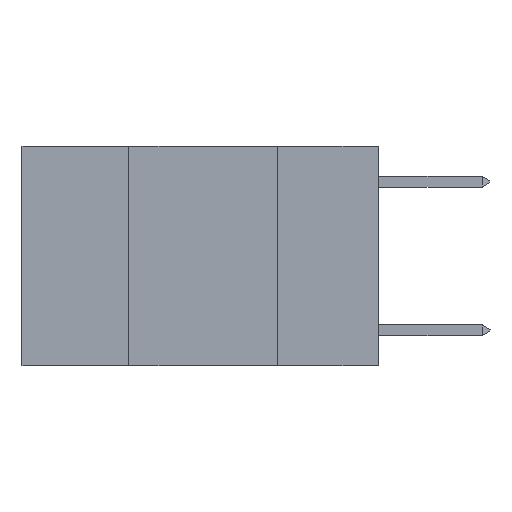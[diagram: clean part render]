
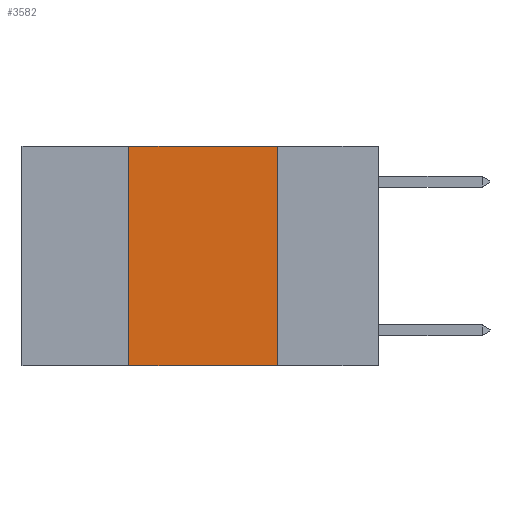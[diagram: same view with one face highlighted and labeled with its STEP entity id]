
A CAD part, left-side view. The second image highlights one B-rep face of the part: STEP entity #3582.
In plain terms, the highlighted planar face has unit normal (-1, 0, 0).
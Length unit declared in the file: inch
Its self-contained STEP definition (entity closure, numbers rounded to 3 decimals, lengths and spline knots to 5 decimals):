
#805 = EDGE_CURVE ( 'NONE', #3752, #4781, #1027, .T. ) ;
#833 = ORIENTED_EDGE ( 'NONE', *, *, #805, .F. ) ;
#1027 = LINE ( 'NONE', #3553, #7129 ) ;
#1480 = LINE ( 'NONE', #6933, #5907 ) ;
#1489 = CARTESIAN_POINT ( 'NONE',  ( 0., 0.17, 0. ) ) ;
#1871 = VECTOR ( 'NONE', #9150, 39.37008 ) ;
#1967 = DIRECTION ( 'NONE',  ( 0., 0., 1. ) ) ;
#2111 = LINE ( 'NONE', #3449, #1871 ) ;
#2640 = LINE ( 'NONE', #1489, #9083 ) ;
#3449 = CARTESIAN_POINT ( 'NONE',  ( 0., 0.6, -0.37 ) ) ;
#3476 = VERTEX_POINT ( 'NONE', #5063 ) ;
#3553 = CARTESIAN_POINT ( 'NONE',  ( 0., 0.6, 0. ) ) ;
#3582 = ADVANCED_FACE ( 'NONE', ( #10185 ), #9226, .F. ) ;
#3752 = VERTEX_POINT ( 'NONE', #4005 ) ;
#4005 = CARTESIAN_POINT ( 'NONE',  ( 0., 0.42, 0. ) ) ;
#4781 = VERTEX_POINT ( 'NONE', #9336 ) ;
#4824 = EDGE_LOOP ( 'NONE', ( #9403, #833, #9914, #4870 ) ) ;
#4870 = ORIENTED_EDGE ( 'NONE', *, *, #6069, .T. ) ;
#5063 = CARTESIAN_POINT ( 'NONE',  ( 0., 0.42, -0.37 ) ) ;
#5273 = EDGE_CURVE ( 'NONE', #4781, #7414, #2640, .T. ) ;
#5336 = DIRECTION ( 'NONE',  ( 0., 0., -1. ) ) ;
#5454 = EDGE_CURVE ( 'NONE', #3476, #3752, #1480, .T. ) ;
#5907 = VECTOR ( 'NONE', #1967, 39.37008 ) ;
#6069 = EDGE_CURVE ( 'NONE', #3476, #7414, #2111, .T. ) ;
#6714 = AXIS2_PLACEMENT_3D ( 'NONE', #8423, #9986, #5336 ) ;
#6933 = CARTESIAN_POINT ( 'NONE',  ( 0., 0.42, 0. ) ) ;
#7129 = VECTOR ( 'NONE', #8106, 39.37008 ) ;
#7265 = DIRECTION ( 'NONE',  ( 0., 0., -1. ) ) ;
#7414 = VERTEX_POINT ( 'NONE', #8835 ) ;
#8106 = DIRECTION ( 'NONE',  ( 0., -1., 0. ) ) ;
#8423 = CARTESIAN_POINT ( 'NONE',  ( 0., 0.6, 0. ) ) ;
#8835 = CARTESIAN_POINT ( 'NONE',  ( 0., 0.17, -0.37 ) ) ;
#9083 = VECTOR ( 'NONE', #7265, 39.37008 ) ;
#9150 = DIRECTION ( 'NONE',  ( 0., -1., 0. ) ) ;
#9226 = PLANE ( 'NONE',  #6714 ) ;
#9336 = CARTESIAN_POINT ( 'NONE',  ( 0., 0.17, 0. ) ) ;
#9403 = ORIENTED_EDGE ( 'NONE', *, *, #5273, .F. ) ;
#9914 = ORIENTED_EDGE ( 'NONE', *, *, #5454, .F. ) ;
#9986 = DIRECTION ( 'NONE',  ( 1., 0., 0. ) ) ;
#10185 = FACE_OUTER_BOUND ( 'NONE', #4824, .T. ) ;
